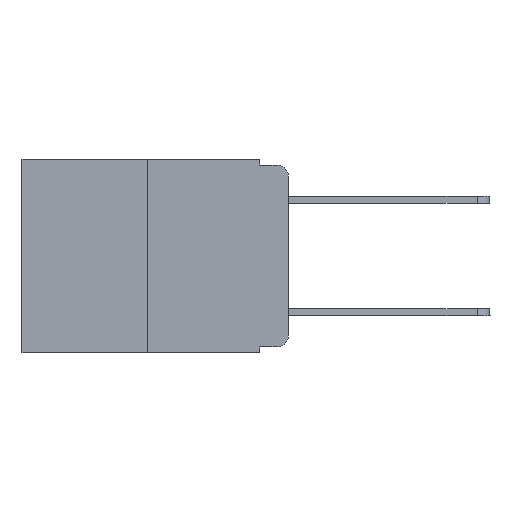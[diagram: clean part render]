
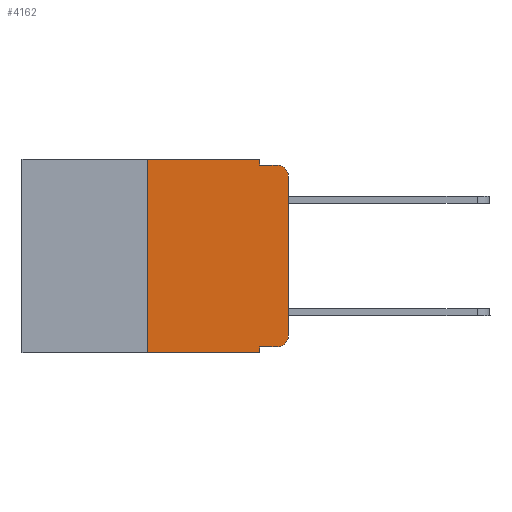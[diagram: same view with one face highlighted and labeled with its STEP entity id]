
A CAD part, left-side view. The second image highlights one B-rep face of the part: STEP entity #4162.
In plain terms, the highlighted planar face has unit normal (-1, 0, 0).
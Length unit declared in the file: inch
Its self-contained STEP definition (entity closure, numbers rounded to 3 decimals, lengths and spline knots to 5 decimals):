
#325 = EDGE_CURVE ( 'NONE', #5759, #13926, #19515, .T. ) ;
#904 = EDGE_CURVE ( 'NONE', #4036, #17561, #10765, .T. ) ;
#1154 = CARTESIAN_POINT ( 'NONE',  ( 0., 0.051, -0.333 ) ) ;
#1262 = LINE ( 'NONE', #10085, #14278 ) ;
#1349 = AXIS2_PLACEMENT_3D ( 'NONE', #21741, #10613, #16067 ) ;
#1424 = EDGE_CURVE ( 'NONE', #23384, #17561, #1262, .T. ) ;
#1704 = CARTESIAN_POINT ( 'NONE',  ( 0., 0.473, -0.343 ) ) ;
#1834 = DIRECTION ( 'NONE',  ( 0., -1., 0. ) ) ;
#1841 = DIRECTION ( 'NONE',  ( 0., 0., -1. ) ) ;
#2015 = EDGE_CURVE ( 'NONE', #10363, #23032, #13547, .T. ) ;
#2248 = VECTOR ( 'NONE', #5190, 39.37008 ) ;
#2514 = EDGE_CURVE ( 'NONE', #20756, #19221, #14690, .T. ) ;
#2530 = ORIENTED_EDGE ( 'NONE', *, *, #904, .T. ) ;
#3438 = CARTESIAN_POINT ( 'NONE',  ( 0., 0., -0.313 ) ) ;
#3642 = EDGE_LOOP ( 'NONE', ( #13777, #10647, #18544, #11372, #4703, #4984, #2530, #7972, #20861, #23581 ) ) ;
#3799 = LINE ( 'NONE', #11604, #8408 ) ;
#4036 = VERTEX_POINT ( 'NONE', #6900 ) ;
#4162 = ADVANCED_FACE ( 'NONE', ( #11134 ), #16721, .F. ) ;
#4275 = CARTESIAN_POINT ( 'NONE',  ( 0., 0.051, -0.343 ) ) ;
#4703 = ORIENTED_EDGE ( 'NONE', *, *, #2514, .F. ) ;
#4878 = LINE ( 'NONE', #6744, #19086 ) ;
#4984 = ORIENTED_EDGE ( 'NONE', *, *, #17605, .F. ) ;
#5190 = DIRECTION ( 'NONE',  ( 0., 0., -1. ) ) ;
#5461 = CARTESIAN_POINT ( 'NONE',  ( 0., 0.473, 0. ) ) ;
#5759 = VERTEX_POINT ( 'NONE', #22248 ) ;
#6744 = CARTESIAN_POINT ( 'NONE',  ( 0., 0., 0. ) ) ;
#6900 = CARTESIAN_POINT ( 'NONE',  ( 0., 0.25, -0.343 ) ) ;
#7876 = DIRECTION ( 'NONE',  ( 0., 0., 1. ) ) ;
#7949 = DIRECTION ( 'NONE',  ( 0., 0., -1. ) ) ;
#7972 = ORIENTED_EDGE ( 'NONE', *, *, #1424, .F. ) ;
#8408 = VECTOR ( 'NONE', #7876, 39.37008 ) ;
#8516 = DIRECTION ( 'NONE',  ( 0., 0., 1. ) ) ;
#9748 = VECTOR ( 'NONE', #1834, 39.37008 ) ;
#10048 = LINE ( 'NONE', #16607, #2248 ) ;
#10085 = CARTESIAN_POINT ( 'NONE',  ( 0., 0.051, 0. ) ) ;
#10168 = EDGE_CURVE ( 'NONE', #23032, #15109, #4878, .T. ) ;
#10302 = VECTOR ( 'NONE', #21376, 39.37008 ) ;
#10363 = VERTEX_POINT ( 'NONE', #16709 ) ;
#10613 = DIRECTION ( 'NONE',  ( -1., 0., 0. ) ) ;
#10647 = ORIENTED_EDGE ( 'NONE', *, *, #18361, .T. ) ;
#10765 = LINE ( 'NONE', #1704, #20400 ) ;
#10770 = EDGE_CURVE ( 'NONE', #19221, #5759, #10048, .T. ) ;
#11134 = FACE_OUTER_BOUND ( 'NONE', #3642, .T. ) ;
#11372 = ORIENTED_EDGE ( 'NONE', *, *, #10770, .F. ) ;
#11604 = CARTESIAN_POINT ( 'NONE',  ( 0., 0.25, 0. ) ) ;
#12308 = CIRCLE ( 'NONE', #1349, 0.02 ) ;
#12902 = CARTESIAN_POINT ( 'NONE',  ( 0., 0.473, 0. ) ) ;
#13216 = LINE ( 'NONE', #1154, #10302 ) ;
#13547 = CIRCLE ( 'NONE', #17967, 0.02 ) ;
#13652 = CARTESIAN_POINT ( 'NONE',  ( 0., 0.051, -0.01 ) ) ;
#13777 = ORIENTED_EDGE ( 'NONE', *, *, #10168, .T. ) ;
#13926 = VERTEX_POINT ( 'NONE', #22181 ) ;
#14278 = VECTOR ( 'NONE', #15934, 39.37008 ) ;
#14690 = LINE ( 'NONE', #12902, #9748 ) ;
#14765 = AXIS2_PLACEMENT_3D ( 'NONE', #5461, #18425, #1841 ) ;
#14889 = CARTESIAN_POINT ( 'NONE',  ( 0., 0.25, 0. ) ) ;
#15109 = VERTEX_POINT ( 'NONE', #16544 ) ;
#15588 = DIRECTION ( 'NONE',  ( -1., 0., 0. ) ) ;
#15934 = DIRECTION ( 'NONE',  ( 0., 0., -1. ) ) ;
#16067 = DIRECTION ( 'NONE',  ( 0., 0., -1. ) ) ;
#16544 = CARTESIAN_POINT ( 'NONE',  ( 0., 0., -0.03 ) ) ;
#16607 = CARTESIAN_POINT ( 'NONE',  ( 0., 0.051, 0. ) ) ;
#16709 = CARTESIAN_POINT ( 'NONE',  ( 0., 0.02, -0.333 ) ) ;
#16721 = PLANE ( 'NONE',  #14765 ) ;
#17144 = EDGE_CURVE ( 'NONE', #23384, #10363, #13216, .T. ) ;
#17206 = VECTOR ( 'NONE', #23051, 39.37008 ) ;
#17561 = VERTEX_POINT ( 'NONE', #4275 ) ;
#17605 = EDGE_CURVE ( 'NONE', #4036, #20756, #3799, .T. ) ;
#17967 = AXIS2_PLACEMENT_3D ( 'NONE', #20927, #15588, #7949 ) ;
#18361 = EDGE_CURVE ( 'NONE', #15109, #13926, #12308, .T. ) ;
#18425 = DIRECTION ( 'NONE',  ( 1., 0., 0. ) ) ;
#18544 = ORIENTED_EDGE ( 'NONE', *, *, #325, .F. ) ;
#19086 = VECTOR ( 'NONE', #8516, 39.37008 ) ;
#19221 = VERTEX_POINT ( 'NONE', #19868 ) ;
#19515 = LINE ( 'NONE', #13652, #17206 ) ;
#19868 = CARTESIAN_POINT ( 'NONE',  ( 0., 0.051, 0. ) ) ;
#20400 = VECTOR ( 'NONE', #22169, 39.37008 ) ;
#20756 = VERTEX_POINT ( 'NONE', #14889 ) ;
#20861 = ORIENTED_EDGE ( 'NONE', *, *, #17144, .T. ) ;
#20927 = CARTESIAN_POINT ( 'NONE',  ( 0., 0.02, -0.313 ) ) ;
#21376 = DIRECTION ( 'NONE',  ( 0., -1., 0. ) ) ;
#21741 = CARTESIAN_POINT ( 'NONE',  ( 0., 0.02, -0.03 ) ) ;
#22169 = DIRECTION ( 'NONE',  ( 0., -1., 0. ) ) ;
#22181 = CARTESIAN_POINT ( 'NONE',  ( 0., 0.02, -0.01 ) ) ;
#22248 = CARTESIAN_POINT ( 'NONE',  ( 0., 0.051, -0.01 ) ) ;
#23032 = VERTEX_POINT ( 'NONE', #3438 ) ;
#23051 = DIRECTION ( 'NONE',  ( 0., -1., 0. ) ) ;
#23384 = VERTEX_POINT ( 'NONE', #23420 ) ;
#23420 = CARTESIAN_POINT ( 'NONE',  ( 0., 0.051, -0.333 ) ) ;
#23581 = ORIENTED_EDGE ( 'NONE', *, *, #2015, .T. ) ;
